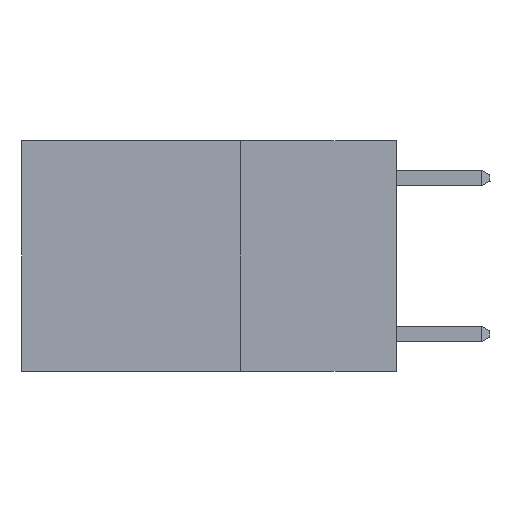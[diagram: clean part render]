
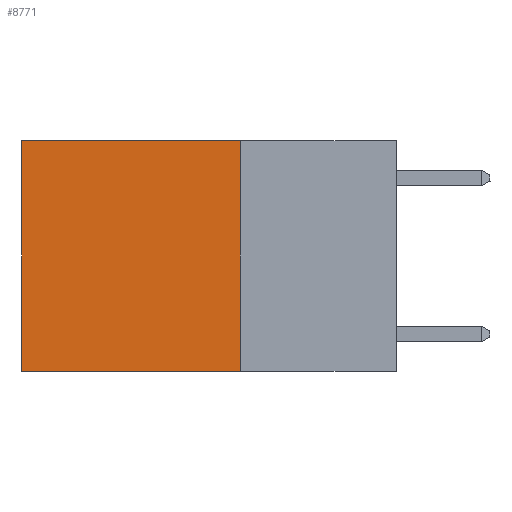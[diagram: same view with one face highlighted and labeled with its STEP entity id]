
A CAD part, left-side view. The second image highlights one B-rep face of the part: STEP entity #8771.
In plain terms, the highlighted planar face has unit normal (-1, 0, 0).
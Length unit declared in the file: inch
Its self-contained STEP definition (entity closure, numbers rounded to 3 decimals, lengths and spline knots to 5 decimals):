
#625 = VECTOR ( 'NONE', #8642, 39.37008 ) ;
#1074 = DIRECTION ( 'NONE',  ( 0., 1., 0. ) ) ;
#1465 = DIRECTION ( 'NONE',  ( 0., 1., 0. ) ) ;
#2332 = EDGE_CURVE ( 'NONE', #3164, #3082, #5022, .T. ) ;
#2562 = EDGE_CURVE ( 'NONE', #11043, #12094, #5258, .T. ) ;
#2881 = CARTESIAN_POINT ( 'NONE',  ( 0.2625, 0.25, 0. ) ) ;
#3082 = VERTEX_POINT ( 'NONE', #14316 ) ;
#3093 = EDGE_CURVE ( 'NONE', #11043, #3164, #18970, .T. ) ;
#3164 = VERTEX_POINT ( 'NONE', #13240 ) ;
#4777 = VECTOR ( 'NONE', #15835, 39.37008 ) ;
#4795 = CARTESIAN_POINT ( 'NONE',  ( 0.2625, 0.6, 0. ) ) ;
#4798 = FACE_OUTER_BOUND ( 'NONE', #13538, .T. ) ;
#4908 = AXIS2_PLACEMENT_3D ( 'NONE', #2881, #17671, #8823 ) ;
#5022 = LINE ( 'NONE', #10004, #12853 ) ;
#5258 = LINE ( 'NONE', #19197, #13092 ) ;
#8641 = LINE ( 'NONE', #9903, #4777 ) ;
#8642 = DIRECTION ( 'NONE',  ( 0., 0., -1. ) ) ;
#8771 = ADVANCED_FACE ( 'NONE', ( #4798 ), #16168, .F. ) ;
#8823 = DIRECTION ( 'NONE',  ( 0., 0., -1. ) ) ;
#9198 = EDGE_CURVE ( 'NONE', #12094, #3082, #8641, .T. ) ;
#9224 = CARTESIAN_POINT ( 'NONE',  ( 0.2625, 0.25, 0. ) ) ;
#9903 = CARTESIAN_POINT ( 'NONE',  ( 0.2625, 0.6, 0. ) ) ;
#10004 = CARTESIAN_POINT ( 'NONE',  ( 0.2625, 0.25, -0.37 ) ) ;
#11043 = VERTEX_POINT ( 'NONE', #9224 ) ;
#12094 = VERTEX_POINT ( 'NONE', #4795 ) ;
#12853 = VECTOR ( 'NONE', #1074, 39.37008 ) ;
#13049 = ORIENTED_EDGE ( 'NONE', *, *, #9198, .T. ) ;
#13092 = VECTOR ( 'NONE', #1465, 39.37008 ) ;
#13240 = CARTESIAN_POINT ( 'NONE',  ( 0.2625, 0.25, -0.37 ) ) ;
#13290 = ORIENTED_EDGE ( 'NONE', *, *, #2332, .F. ) ;
#13538 = EDGE_LOOP ( 'NONE', ( #13049, #13290, #15076, #15423 ) ) ;
#14316 = CARTESIAN_POINT ( 'NONE',  ( 0.2625, 0.6, -0.37 ) ) ;
#15076 = ORIENTED_EDGE ( 'NONE', *, *, #3093, .F. ) ;
#15423 = ORIENTED_EDGE ( 'NONE', *, *, #2562, .T. ) ;
#15731 = CARTESIAN_POINT ( 'NONE',  ( 0.2625, 0.25, 0. ) ) ;
#15835 = DIRECTION ( 'NONE',  ( 0., 0., -1. ) ) ;
#16168 = PLANE ( 'NONE',  #4908 ) ;
#17671 = DIRECTION ( 'NONE',  ( 1., 0., 0. ) ) ;
#18970 = LINE ( 'NONE', #15731, #625 ) ;
#19197 = CARTESIAN_POINT ( 'NONE',  ( 0.2625, 0.25, 0. ) ) ;
